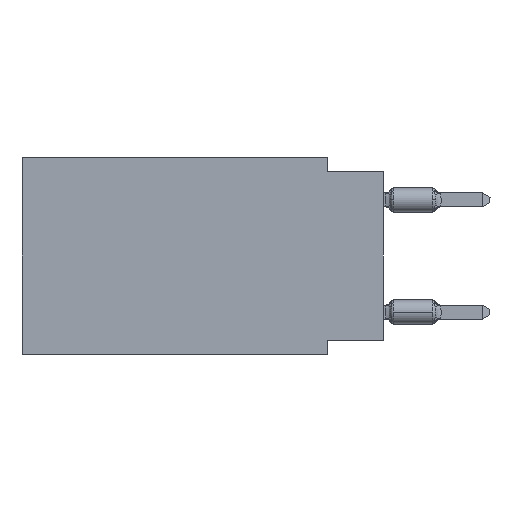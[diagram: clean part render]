
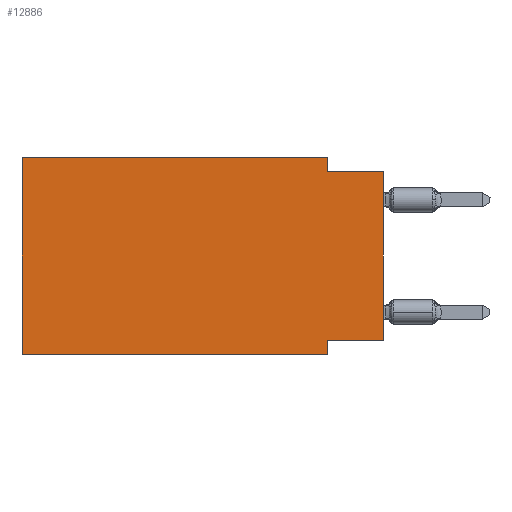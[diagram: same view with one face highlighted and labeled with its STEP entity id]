
A CAD part, left-side view. The second image highlights one B-rep face of the part: STEP entity #12886.
In plain terms, the highlighted planar face has unit normal (-1, 0, 0).
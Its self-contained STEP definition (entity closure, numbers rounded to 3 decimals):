
#620 = ORIENTED_EDGE ( 'NONE', *, *, #50712, .F. ) ;
#792 = LINE ( 'NONE', #17336, #46166 ) ;
#2076 = DIRECTION ( 'NONE',  ( 0., 0., 1. ) ) ;
#2336 = CARTESIAN_POINT ( 'NONE',  ( 0., 16.383, 0. ) ) ;
#3187 = VERTEX_POINT ( 'NONE', #3900 ) ;
#3900 = CARTESIAN_POINT ( 'NONE',  ( 0., 0., -8.255 ) ) ;
#4403 = VECTOR ( 'NONE', #46950, 1000. ) ;
#4973 = ORIENTED_EDGE ( 'NONE', *, *, #39322, .F. ) ;
#5173 = EDGE_CURVE ( 'NONE', #3187, #6830, #21661, .T. ) ;
#5214 = LINE ( 'NONE', #10095, #38346 ) ;
#5543 = CARTESIAN_POINT ( 'NONE',  ( 0., 16.383, -8.89 ) ) ;
#6161 = CARTESIAN_POINT ( 'NONE',  ( 0., 2.54, -8.255 ) ) ;
#6341 = EDGE_CURVE ( 'NONE', #35811, #47814, #792, .T. ) ;
#6830 = VERTEX_POINT ( 'NONE', #6161 ) ;
#8107 = DIRECTION ( 'NONE',  ( 0., 0., -1. ) ) ;
#8959 = EDGE_CURVE ( 'NONE', #35811, #40588, #46885, .T. ) ;
#10095 = CARTESIAN_POINT ( 'NONE',  ( 0., 0., 0. ) ) ;
#11938 = CARTESIAN_POINT ( 'NONE',  ( 0., 0., -0.635 ) ) ;
#12449 = LINE ( 'NONE', #24915, #30450 ) ;
#12886 = ADVANCED_FACE ( 'NONE', ( #16350 ), #45675, .F. ) ;
#13564 = DIRECTION ( 'NONE',  ( 0., -1., 0. ) ) ;
#14834 = DIRECTION ( 'NONE',  ( 0., 0., -1. ) ) ;
#16350 = FACE_OUTER_BOUND ( 'NONE', #53417, .T. ) ;
#16513 = ORIENTED_EDGE ( 'NONE', *, *, #5173, .F. ) ;
#16760 = CARTESIAN_POINT ( 'NONE',  ( 0., 2.54, -8.89 ) ) ;
#17010 = CARTESIAN_POINT ( 'NONE',  ( 0., 16.383, 0. ) ) ;
#17135 = DIRECTION ( 'NONE',  ( 1., 0., 0. ) ) ;
#17158 = VECTOR ( 'NONE', #2076, 1000. ) ;
#17336 = CARTESIAN_POINT ( 'NONE',  ( 0., 16.383, -8.89 ) ) ;
#21347 = LINE ( 'NONE', #16760, #47990 ) ;
#21558 = VERTEX_POINT ( 'NONE', #42563 ) ;
#21661 = LINE ( 'NONE', #30355, #4403 ) ;
#22520 = AXIS2_PLACEMENT_3D ( 'NONE', #46210, #17135, #32927 ) ;
#23496 = CARTESIAN_POINT ( 'NONE',  ( 0., 2.54, 0. ) ) ;
#24096 = DIRECTION ( 'NONE',  ( 0., -1., 0. ) ) ;
#24915 = CARTESIAN_POINT ( 'NONE',  ( 0., 0., -0.635 ) ) ;
#25440 = ORIENTED_EDGE ( 'NONE', *, *, #39076, .F. ) ;
#27774 = CARTESIAN_POINT ( 'NONE',  ( 0., 2.54, 0. ) ) ;
#28550 = ORIENTED_EDGE ( 'NONE', *, *, #6341, .T. ) ;
#29538 = VECTOR ( 'NONE', #14834, 1000. ) ;
#30355 = CARTESIAN_POINT ( 'NONE',  ( 0., 0., -8.255 ) ) ;
#30450 = VECTOR ( 'NONE', #24096, 1000. ) ;
#32067 = ORIENTED_EDGE ( 'NONE', *, *, #42446, .T. ) ;
#32608 = ORIENTED_EDGE ( 'NONE', *, *, #40866, .F. ) ;
#32927 = DIRECTION ( 'NONE',  ( 0., 0., -1. ) ) ;
#33909 = DIRECTION ( 'NONE',  ( 0., -1., 0. ) ) ;
#34503 = DIRECTION ( 'NONE',  ( 0., 0., 1. ) ) ;
#35032 = ORIENTED_EDGE ( 'NONE', *, *, #8959, .F. ) ;
#35455 = LINE ( 'NONE', #23496, #29538 ) ;
#35811 = VERTEX_POINT ( 'NONE', #5543 ) ;
#38346 = VECTOR ( 'NONE', #34503, 1000. ) ;
#38797 = CARTESIAN_POINT ( 'NONE',  ( 0., 16.383, 0. ) ) ;
#39076 = EDGE_CURVE ( 'NONE', #40588, #46783, #42067, .T. ) ;
#39322 = EDGE_CURVE ( 'NONE', #21558, #41564, #12449, .T. ) ;
#40588 = VERTEX_POINT ( 'NONE', #17010 ) ;
#40866 = EDGE_CURVE ( 'NONE', #46783, #21558, #35455, .T. ) ;
#41564 = VERTEX_POINT ( 'NONE', #11938 ) ;
#42067 = LINE ( 'NONE', #38797, #47766 ) ;
#42446 = EDGE_CURVE ( 'NONE', #3187, #41564, #5214, .T. ) ;
#42563 = CARTESIAN_POINT ( 'NONE',  ( 0., 2.54, -0.635 ) ) ;
#45675 = PLANE ( 'NONE',  #22520 ) ;
#46166 = VECTOR ( 'NONE', #33909, 1000. ) ;
#46210 = CARTESIAN_POINT ( 'NONE',  ( 0., 16.383, 0. ) ) ;
#46783 = VERTEX_POINT ( 'NONE', #27774 ) ;
#46885 = LINE ( 'NONE', #2336, #17158 ) ;
#46950 = DIRECTION ( 'NONE',  ( 0., 1., 0. ) ) ;
#47766 = VECTOR ( 'NONE', #13564, 1000. ) ;
#47814 = VERTEX_POINT ( 'NONE', #50214 ) ;
#47990 = VECTOR ( 'NONE', #8107, 1000. ) ;
#50214 = CARTESIAN_POINT ( 'NONE',  ( 0., 2.54, -8.89 ) ) ;
#50712 = EDGE_CURVE ( 'NONE', #6830, #47814, #21347, .T. ) ;
#53417 = EDGE_LOOP ( 'NONE', ( #32067, #4973, #32608, #25440, #35032, #28550, #620, #16513 ) ) ;
